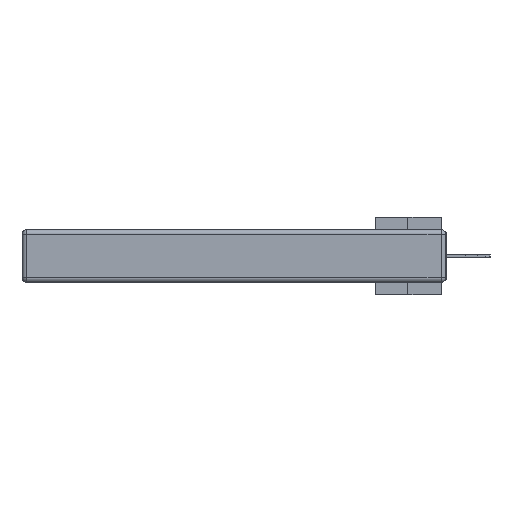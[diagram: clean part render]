
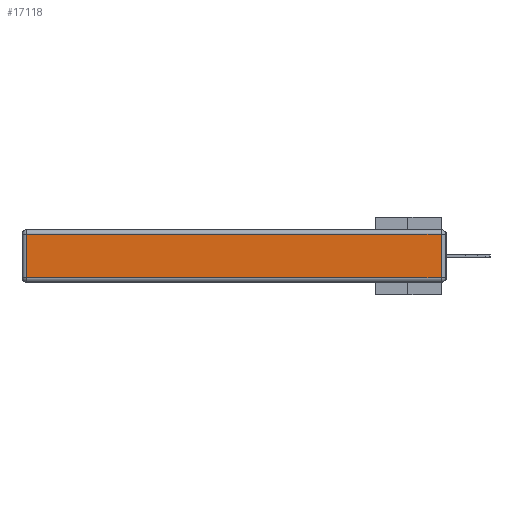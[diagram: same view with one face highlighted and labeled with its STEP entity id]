
A CAD part, left-side view. The second image highlights one B-rep face of the part: STEP entity #17118.
In plain terms, the highlighted planar face has unit normal (-1, 0, 0).
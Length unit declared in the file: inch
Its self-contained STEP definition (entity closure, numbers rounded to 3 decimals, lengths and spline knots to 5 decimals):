
#1655 = AXIS2_PLACEMENT_3D ( 'NONE', #4472, #33216, #8073 ) ;
#3395 = EDGE_CURVE ( 'NONE', #16621, #21253, #4730, .T. ) ;
#4472 = CARTESIAN_POINT ( 'NONE',  ( 0., 0., -0.343 ) ) ;
#4730 = LINE ( 'NONE', #30715, #13702 ) ;
#5297 = CARTESIAN_POINT ( 'NONE',  ( 0., 2.72, -0.343 ) ) ;
#5862 = CARTESIAN_POINT ( 'NONE',  ( 0., 0.03, -0.313 ) ) ;
#7010 = ORIENTED_EDGE ( 'NONE', *, *, #34790, .T. ) ;
#8073 = DIRECTION ( 'NONE',  ( 0., 0., 1. ) ) ;
#8329 = DIRECTION ( 'NONE',  ( 0., -1., 0. ) ) ;
#11101 = CARTESIAN_POINT ( 'NONE',  ( 0., 0., -0.313 ) ) ;
#13702 = VECTOR ( 'NONE', #34734, 39.37008 ) ;
#14945 = VERTEX_POINT ( 'NONE', #22485 ) ;
#15304 = DIRECTION ( 'NONE',  ( 0., 0., -1. ) ) ;
#16621 = VERTEX_POINT ( 'NONE', #5862 ) ;
#17118 = ADVANCED_FACE ( 'NONE', ( #33623 ), #20847, .T. ) ;
#18183 = VECTOR ( 'NONE', #8329, 39.37008 ) ;
#18916 = DIRECTION ( 'NONE',  ( 0., 1., 0. ) ) ;
#20847 = PLANE ( 'NONE',  #1655 ) ;
#21253 = VERTEX_POINT ( 'NONE', #23797 ) ;
#21692 = EDGE_CURVE ( 'NONE', #41489, #16621, #27702, .T. ) ;
#22208 = VECTOR ( 'NONE', #15304, 39.37008 ) ;
#22485 = CARTESIAN_POINT ( 'NONE',  ( 0., 2.72, -0.03 ) ) ;
#23797 = CARTESIAN_POINT ( 'NONE',  ( 0., 0.03, -0.03 ) ) ;
#24642 = EDGE_CURVE ( 'NONE', #21253, #14945, #35973, .T. ) ;
#25296 = VECTOR ( 'NONE', #18916, 39.37008 ) ;
#27702 = LINE ( 'NONE', #11101, #18183 ) ;
#30715 = CARTESIAN_POINT ( 'NONE',  ( 0., 0.03, -0.343 ) ) ;
#31062 = LINE ( 'NONE', #5297, #22208 ) ;
#32344 = ORIENTED_EDGE ( 'NONE', *, *, #24642, .T. ) ;
#32944 = CARTESIAN_POINT ( 'NONE',  ( 0., 2.72, -0.313 ) ) ;
#33216 = DIRECTION ( 'NONE',  ( -1., 0., 0. ) ) ;
#33623 = FACE_OUTER_BOUND ( 'NONE', #38291, .T. ) ;
#34160 = ORIENTED_EDGE ( 'NONE', *, *, #3395, .T. ) ;
#34505 = ORIENTED_EDGE ( 'NONE', *, *, #21692, .T. ) ;
#34734 = DIRECTION ( 'NONE',  ( 0., 0., 1. ) ) ;
#34790 = EDGE_CURVE ( 'NONE', #14945, #41489, #31062, .T. ) ;
#35973 = LINE ( 'NONE', #38968, #25296 ) ;
#38291 = EDGE_LOOP ( 'NONE', ( #34505, #34160, #32344, #7010 ) ) ;
#38968 = CARTESIAN_POINT ( 'NONE',  ( 0., 2.75, -0.03 ) ) ;
#41489 = VERTEX_POINT ( 'NONE', #32944 ) ;
